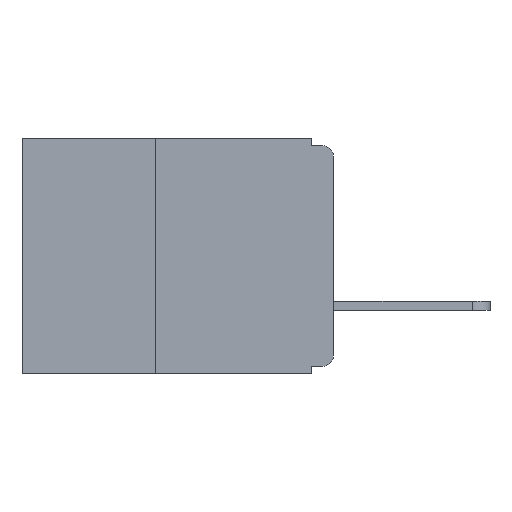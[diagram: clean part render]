
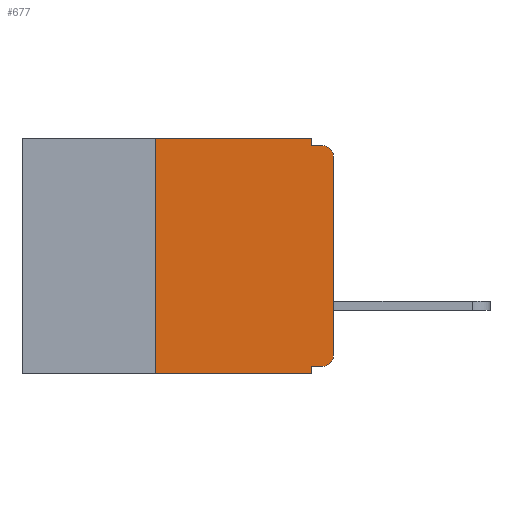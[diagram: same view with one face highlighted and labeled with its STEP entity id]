
A CAD part, left-side view. The second image highlights one B-rep face of the part: STEP entity #677.
In plain terms, the highlighted planar face has unit normal (-1, 0, 0).
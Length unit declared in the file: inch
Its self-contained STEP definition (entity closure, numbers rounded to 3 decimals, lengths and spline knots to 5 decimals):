
#298 = ORIENTED_EDGE ( 'NONE', *, *, #4193, .T. ) ;
#347 = LINE ( 'NONE', #1397, #2813 ) ;
#575 = VERTEX_POINT ( 'NONE', #11963 ) ;
#597 = DIRECTION ( 'NONE',  ( 0., 0., 1. ) ) ;
#677 = ADVANCED_FACE ( 'NONE', ( #2269 ), #4178, .F. ) ;
#712 = CARTESIAN_POINT ( 'NONE',  ( 0., 0.031, -0.33 ) ) ;
#1193 = DIRECTION ( 'NONE',  ( 0., 0., -1. ) ) ;
#1288 = CARTESIAN_POINT ( 'NONE',  ( 0., 0.437, 0. ) ) ;
#1299 = VECTOR ( 'NONE', #8998, 39.37008 ) ;
#1328 = CARTESIAN_POINT ( 'NONE',  ( 0., 0.25, -0.33 ) ) ;
#1333 = CARTESIAN_POINT ( 'NONE',  ( 0., 0.031, -0.01 ) ) ;
#1397 = CARTESIAN_POINT ( 'NONE',  ( 0., 0., 0. ) ) ;
#1441 = LINE ( 'NONE', #5963, #1299 ) ;
#2131 = CARTESIAN_POINT ( 'NONE',  ( 0., 0., -0.025 ) ) ;
#2269 = FACE_OUTER_BOUND ( 'NONE', #8839, .T. ) ;
#2411 = CARTESIAN_POINT ( 'NONE',  ( 0., 0.015, -0.01 ) ) ;
#2412 = VECTOR ( 'NONE', #6599, 39.37008 ) ;
#2435 = EDGE_CURVE ( 'NONE', #6050, #7737, #347, .T. ) ;
#2557 = DIRECTION ( 'NONE',  ( 0., -1., 0. ) ) ;
#2656 = CARTESIAN_POINT ( 'NONE',  ( 0., 0.031, -0.33 ) ) ;
#2813 = VECTOR ( 'NONE', #8424, 39.37008 ) ;
#2910 = VECTOR ( 'NONE', #10877, 39.37008 ) ;
#3011 = VERTEX_POINT ( 'NONE', #4437 ) ;
#3077 = ORIENTED_EDGE ( 'NONE', *, *, #4957, .F. ) ;
#3146 = CARTESIAN_POINT ( 'NONE',  ( 0., 0.031, 0. ) ) ;
#3147 = ORIENTED_EDGE ( 'NONE', *, *, #6085, .T. ) ;
#3476 = VERTEX_POINT ( 'NONE', #4686 ) ;
#3599 = ORIENTED_EDGE ( 'NONE', *, *, #8899, .T. ) ;
#3951 = DIRECTION ( 'NONE',  ( -1., 0., 0. ) ) ;
#4178 = PLANE ( 'NONE',  #12524 ) ;
#4186 = AXIS2_PLACEMENT_3D ( 'NONE', #7037, #3951, #6869 ) ;
#4193 = EDGE_CURVE ( 'NONE', #11387, #6324, #10735, .T. ) ;
#4228 = DIRECTION ( 'NONE',  ( 0., -1., 0. ) ) ;
#4437 = CARTESIAN_POINT ( 'NONE',  ( 0., 0.031, -0.32 ) ) ;
#4686 = CARTESIAN_POINT ( 'NONE',  ( 0., 0.015, -0.32 ) ) ;
#4957 = EDGE_CURVE ( 'NONE', #11387, #575, #12569, .T. ) ;
#5476 = LINE ( 'NONE', #8326, #9706 ) ;
#5507 = EDGE_CURVE ( 'NONE', #8091, #7071, #10867, .T. ) ;
#5634 = ORIENTED_EDGE ( 'NONE', *, *, #2435, .T. ) ;
#5686 = ORIENTED_EDGE ( 'NONE', *, *, #9151, .F. ) ;
#5963 = CARTESIAN_POINT ( 'NONE',  ( 0., 0., -0.32 ) ) ;
#6016 = CIRCLE ( 'NONE', #10383, 0.015 ) ;
#6050 = VERTEX_POINT ( 'NONE', #7961 ) ;
#6085 = EDGE_CURVE ( 'NONE', #3476, #6050, #6016, .T. ) ;
#6108 = DIRECTION ( 'NONE',  ( -1., 0., 0. ) ) ;
#6142 = CARTESIAN_POINT ( 'NONE',  ( 0., 0.015, -0.305 ) ) ;
#6324 = VERTEX_POINT ( 'NONE', #712 ) ;
#6358 = VECTOR ( 'NONE', #2557, 39.37008 ) ;
#6437 = CARTESIAN_POINT ( 'NONE',  ( 0., 0.031, 0. ) ) ;
#6511 = VECTOR ( 'NONE', #10281, 39.37008 ) ;
#6599 = DIRECTION ( 'NONE',  ( 0., 0., -1. ) ) ;
#6767 = EDGE_CURVE ( 'NONE', #3011, #6324, #9894, .T. ) ;
#6869 = DIRECTION ( 'NONE',  ( 0., 0., -1. ) ) ;
#7037 = CARTESIAN_POINT ( 'NONE',  ( 0., 0.015, -0.025 ) ) ;
#7071 = VERTEX_POINT ( 'NONE', #1333 ) ;
#7499 = VERTEX_POINT ( 'NONE', #2411 ) ;
#7601 = LINE ( 'NONE', #10924, #2910 ) ;
#7652 = EDGE_CURVE ( 'NONE', #3476, #3011, #1441, .T. ) ;
#7719 = CARTESIAN_POINT ( 'NONE',  ( 0., 0.437, -0.33 ) ) ;
#7737 = VERTEX_POINT ( 'NONE', #2131 ) ;
#7911 = ORIENTED_EDGE ( 'NONE', *, *, #5507, .F. ) ;
#7961 = CARTESIAN_POINT ( 'NONE',  ( 0., 0., -0.305 ) ) ;
#8091 = VERTEX_POINT ( 'NONE', #6437 ) ;
#8139 = DIRECTION ( 'NONE',  ( 1., 0., 0. ) ) ;
#8326 = CARTESIAN_POINT ( 'NONE',  ( 0., 0.437, 0. ) ) ;
#8424 = DIRECTION ( 'NONE',  ( 0., 0., 1. ) ) ;
#8455 = ORIENTED_EDGE ( 'NONE', *, *, #6767, .F. ) ;
#8839 = EDGE_LOOP ( 'NONE', ( #5634, #3599, #5686, #7911, #12567, #3077, #298, #8455, #12826, #3147 ) ) ;
#8899 = EDGE_CURVE ( 'NONE', #7737, #7499, #9019, .T. ) ;
#8998 = DIRECTION ( 'NONE',  ( 0., 1., 0. ) ) ;
#9019 = CIRCLE ( 'NONE', #4186, 0.015 ) ;
#9098 = DIRECTION ( 'NONE',  ( 0., 0., -1. ) ) ;
#9151 = EDGE_CURVE ( 'NONE', #7071, #7499, #7601, .T. ) ;
#9706 = VECTOR ( 'NONE', #4228, 39.37008 ) ;
#9894 = LINE ( 'NONE', #2656, #2412 ) ;
#10281 = DIRECTION ( 'NONE',  ( 0., 0., -1. ) ) ;
#10383 = AXIS2_PLACEMENT_3D ( 'NONE', #6142, #6108, #1193 ) ;
#10735 = LINE ( 'NONE', #7719, #6358 ) ;
#10867 = LINE ( 'NONE', #3146, #6511 ) ;
#10877 = DIRECTION ( 'NONE',  ( 0., -1., 0. ) ) ;
#10924 = CARTESIAN_POINT ( 'NONE',  ( 0., 0., -0.01 ) ) ;
#11387 = VERTEX_POINT ( 'NONE', #1328 ) ;
#11497 = CARTESIAN_POINT ( 'NONE',  ( 0., 0.25, -0.33 ) ) ;
#11503 = VECTOR ( 'NONE', #597, 39.37008 ) ;
#11902 = EDGE_CURVE ( 'NONE', #575, #8091, #5476, .T. ) ;
#11963 = CARTESIAN_POINT ( 'NONE',  ( 0., 0.25, 0. ) ) ;
#12524 = AXIS2_PLACEMENT_3D ( 'NONE', #1288, #8139, #9098 ) ;
#12567 = ORIENTED_EDGE ( 'NONE', *, *, #11902, .F. ) ;
#12569 = LINE ( 'NONE', #11497, #11503 ) ;
#12826 = ORIENTED_EDGE ( 'NONE', *, *, #7652, .F. ) ;
